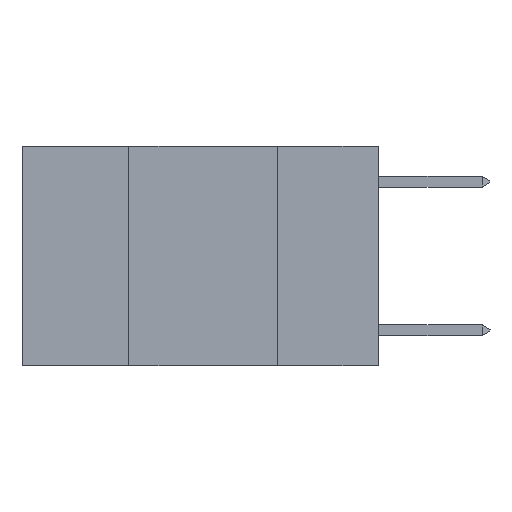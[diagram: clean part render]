
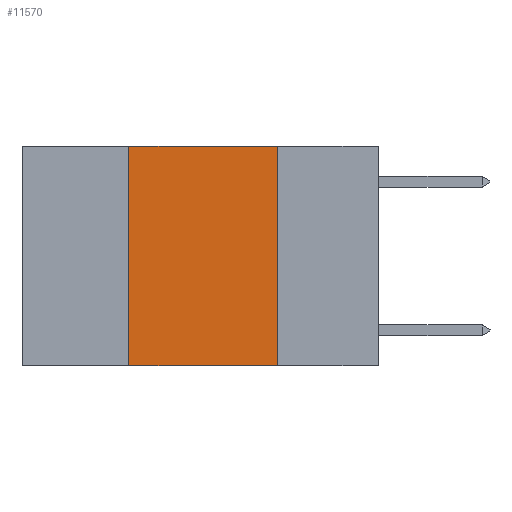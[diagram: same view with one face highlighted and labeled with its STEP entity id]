
A CAD part, left-side view. The second image highlights one B-rep face of the part: STEP entity #11570.
In plain terms, the highlighted planar face has unit normal (-1, 0, 0).
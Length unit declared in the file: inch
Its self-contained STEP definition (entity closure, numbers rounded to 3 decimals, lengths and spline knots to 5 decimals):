
#180 = ORIENTED_EDGE ( 'NONE', *, *, #21573, .F. ) ;
#255 = EDGE_CURVE ( 'NONE', #6991, #13732, #26325, .T. ) ;
#1173 = ORIENTED_EDGE ( 'NONE', *, *, #255, .F. ) ;
#1987 = VECTOR ( 'NONE', #17186, 39.37008 ) ;
#2077 = LINE ( 'NONE', #17755, #1987 ) ;
#2175 = ORIENTED_EDGE ( 'NONE', *, *, #7048, .F. ) ;
#3623 = VECTOR ( 'NONE', #26243, 39.37008 ) ;
#6991 = VERTEX_POINT ( 'NONE', #20233 ) ;
#7048 = EDGE_CURVE ( 'NONE', #13732, #25051, #2077, .T. ) ;
#7259 = VECTOR ( 'NONE', #8653, 39.37008 ) ;
#8653 = DIRECTION ( 'NONE',  ( 0., -1., 0. ) ) ;
#8719 = CARTESIAN_POINT ( 'NONE',  ( 0., 0.42, -0.37 ) ) ;
#11420 = PLANE ( 'NONE',  #13641 ) ;
#11570 = ADVANCED_FACE ( 'NONE', ( #13572 ), #11420, .F. ) ;
#11710 = DIRECTION ( 'NONE',  ( 0., -1., 0. ) ) ;
#11937 = CARTESIAN_POINT ( 'NONE',  ( 0., 0.42, 0. ) ) ;
#12010 = CARTESIAN_POINT ( 'NONE',  ( 0., 0.6, 0. ) ) ;
#13381 = LINE ( 'NONE', #11937, #3623 ) ;
#13428 = CARTESIAN_POINT ( 'NONE',  ( 0., 0.6, 0. ) ) ;
#13517 = DIRECTION ( 'NONE',  ( 0., 0., -1. ) ) ;
#13572 = FACE_OUTER_BOUND ( 'NONE', #20451, .T. ) ;
#13641 = AXIS2_PLACEMENT_3D ( 'NONE', #13428, #25703, #13517 ) ;
#13732 = VERTEX_POINT ( 'NONE', #15217 ) ;
#15217 = CARTESIAN_POINT ( 'NONE',  ( 0., 0.17, 0. ) ) ;
#17186 = DIRECTION ( 'NONE',  ( 0., 0., -1. ) ) ;
#17755 = CARTESIAN_POINT ( 'NONE',  ( 0., 0.17, 0. ) ) ;
#17798 = LINE ( 'NONE', #19073, #7259 ) ;
#19039 = CARTESIAN_POINT ( 'NONE',  ( 0., 0.17, -0.37 ) ) ;
#19073 = CARTESIAN_POINT ( 'NONE',  ( 0., 0.6, -0.37 ) ) ;
#20233 = CARTESIAN_POINT ( 'NONE',  ( 0., 0.42, 0. ) ) ;
#20451 = EDGE_LOOP ( 'NONE', ( #2175, #1173, #180, #26695 ) ) ;
#21573 = EDGE_CURVE ( 'NONE', #25063, #6991, #13381, .T. ) ;
#25051 = VERTEX_POINT ( 'NONE', #19039 ) ;
#25063 = VERTEX_POINT ( 'NONE', #8719 ) ;
#25703 = DIRECTION ( 'NONE',  ( 1., 0., 0. ) ) ;
#26217 = VECTOR ( 'NONE', #11710, 39.37008 ) ;
#26243 = DIRECTION ( 'NONE',  ( 0., 0., 1. ) ) ;
#26325 = LINE ( 'NONE', #12010, #26217 ) ;
#26373 = EDGE_CURVE ( 'NONE', #25063, #25051, #17798, .T. ) ;
#26695 = ORIENTED_EDGE ( 'NONE', *, *, #26373, .T. ) ;
